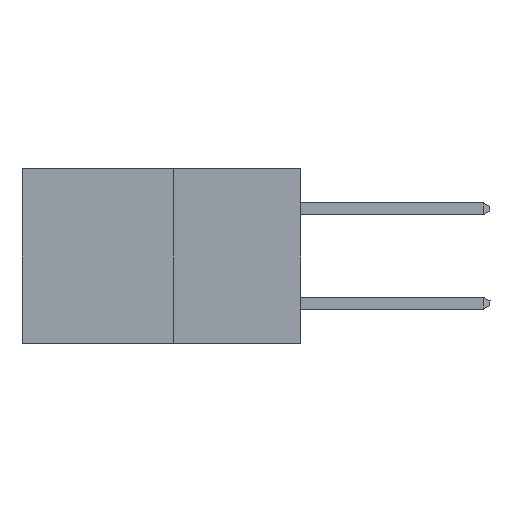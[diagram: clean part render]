
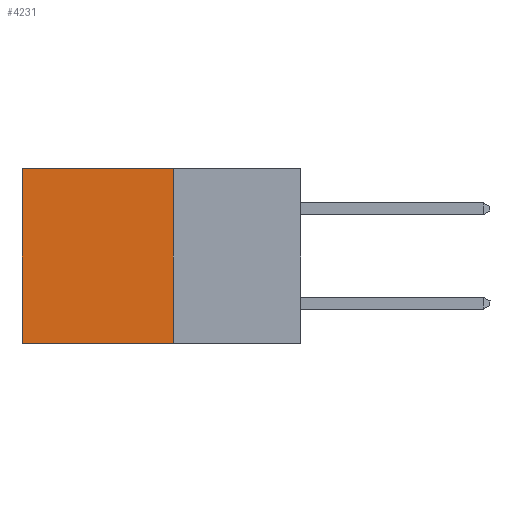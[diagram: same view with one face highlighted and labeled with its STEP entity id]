
A CAD part, left-side view. The second image highlights one B-rep face of the part: STEP entity #4231.
In plain terms, the highlighted planar face has unit normal (-1, 0, 0).
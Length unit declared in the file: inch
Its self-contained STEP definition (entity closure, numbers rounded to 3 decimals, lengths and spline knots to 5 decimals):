
#2454 = DIRECTION ( 'NONE',  ( 0., 1., 0. ) ) ;
#3271 = EDGE_CURVE ( 'NONE', #19093, #9529, #21156, .T. ) ;
#3502 = ORIENTED_EDGE ( 'NONE', *, *, #3271, .F. ) ;
#3705 = CARTESIAN_POINT ( 'NONE',  ( 0.277, 0.27, 0. ) ) ;
#4231 = ADVANCED_FACE ( 'NONE', ( #6456 ), #26013, .F. ) ;
#6456 = FACE_OUTER_BOUND ( 'NONE', #21549, .T. ) ;
#6657 = DIRECTION ( 'NONE',  ( 0., 1., 0. ) ) ;
#6720 = CARTESIAN_POINT ( 'NONE',  ( 0.277, 0.59, -0.37 ) ) ;
#8088 = LINE ( 'NONE', #6720, #29197 ) ;
#9529 = VERTEX_POINT ( 'NONE', #17851 ) ;
#10957 = ORIENTED_EDGE ( 'NONE', *, *, #32499, .T. ) ;
#12274 = DIRECTION ( 'NONE',  ( 0., 0., -1. ) ) ;
#12314 = DIRECTION ( 'NONE',  ( 1., 0., 0. ) ) ;
#13476 = ORIENTED_EDGE ( 'NONE', *, *, #26483, .F. ) ;
#14298 = CARTESIAN_POINT ( 'NONE',  ( 0.277, 0.27, -0.37 ) ) ;
#14369 = ORIENTED_EDGE ( 'NONE', *, *, #26805, .T. ) ;
#15756 = VERTEX_POINT ( 'NONE', #21170 ) ;
#15872 = VERTEX_POINT ( 'NONE', #18866 ) ;
#16071 = CARTESIAN_POINT ( 'NONE',  ( 0.277, 0.27, 0. ) ) ;
#17547 = LINE ( 'NONE', #19062, #24855 ) ;
#17851 = CARTESIAN_POINT ( 'NONE',  ( 0.277, 0.27, -0.37 ) ) ;
#18866 = CARTESIAN_POINT ( 'NONE',  ( 0.277, 0.59, -0.37 ) ) ;
#19062 = CARTESIAN_POINT ( 'NONE',  ( 0.277, 0.27, -0.37 ) ) ;
#19093 = VERTEX_POINT ( 'NONE', #16071 ) ;
#20969 = LINE ( 'NONE', #3705, #27445 ) ;
#21156 = LINE ( 'NONE', #14298, #34070 ) ;
#21170 = CARTESIAN_POINT ( 'NONE',  ( 0.277, 0.59, 0. ) ) ;
#21549 = EDGE_LOOP ( 'NONE', ( #10957, #13476, #3502, #14369 ) ) ;
#23225 = CARTESIAN_POINT ( 'NONE',  ( 0.277, 0.27, -0.37 ) ) ;
#23961 = AXIS2_PLACEMENT_3D ( 'NONE', #23225, #12314, #31557 ) ;
#24855 = VECTOR ( 'NONE', #2454, 39.37008 ) ;
#25199 = DIRECTION ( 'NONE',  ( 0., 0., -1. ) ) ;
#26013 = PLANE ( 'NONE',  #23961 ) ;
#26483 = EDGE_CURVE ( 'NONE', #9529, #15872, #17547, .T. ) ;
#26805 = EDGE_CURVE ( 'NONE', #19093, #15756, #20969, .T. ) ;
#27445 = VECTOR ( 'NONE', #6657, 39.37008 ) ;
#29197 = VECTOR ( 'NONE', #12274, 39.37008 ) ;
#31557 = DIRECTION ( 'NONE',  ( 0., 0., -1. ) ) ;
#32499 = EDGE_CURVE ( 'NONE', #15756, #15872, #8088, .T. ) ;
#34070 = VECTOR ( 'NONE', #25199, 39.37008 ) ;
